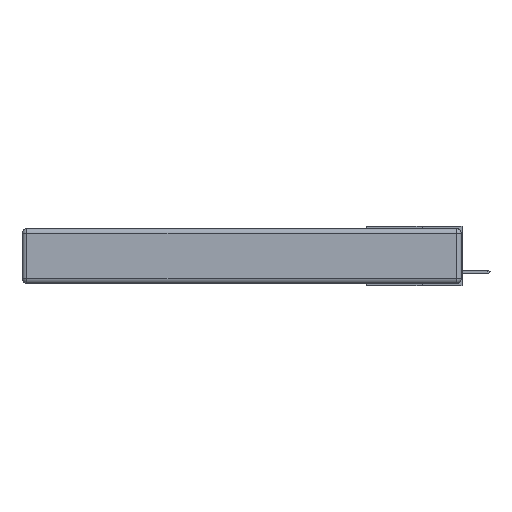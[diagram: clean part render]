
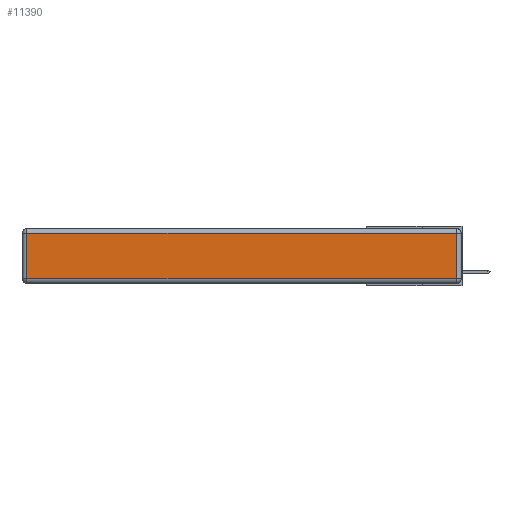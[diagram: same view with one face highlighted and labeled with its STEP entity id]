
A CAD part, left-side view. The second image highlights one B-rep face of the part: STEP entity #11390.
In plain terms, the highlighted planar face has unit normal (-1, 0, 0).
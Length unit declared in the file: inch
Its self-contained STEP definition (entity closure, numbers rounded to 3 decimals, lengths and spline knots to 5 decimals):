
#704 = CARTESIAN_POINT ( 'NONE',  ( 0., 0., -0.313 ) ) ;
#981 = VECTOR ( 'NONE', #4588, 39.37008 ) ;
#1590 = ORIENTED_EDGE ( 'NONE', *, *, #9891, .T. ) ;
#2071 = DIRECTION ( 'NONE',  ( 0., 0., 1. ) ) ;
#2267 = CARTESIAN_POINT ( 'NONE',  ( 0., 0., -0.343 ) ) ;
#2925 = VECTOR ( 'NONE', #2071, 39.37008 ) ;
#3695 = PLANE ( 'NONE',  #12956 ) ;
#4060 = EDGE_CURVE ( 'NONE', #6856, #14150, #15080, .T. ) ;
#4332 = CARTESIAN_POINT ( 'NONE',  ( 0., 0.03, -0.313 ) ) ;
#4337 = VERTEX_POINT ( 'NONE', #4332 ) ;
#4588 = DIRECTION ( 'NONE',  ( 0., 0., -1. ) ) ;
#5303 = DIRECTION ( 'NONE',  ( 0., 1., 0. ) ) ;
#6033 = VERTEX_POINT ( 'NONE', #11285 ) ;
#6305 = CARTESIAN_POINT ( 'NONE',  ( 0., 2.72, -0.343 ) ) ;
#6407 = VECTOR ( 'NONE', #5303, 39.37008 ) ;
#6719 = CARTESIAN_POINT ( 'NONE',  ( 0., 0.03, -0.343 ) ) ;
#6856 = VERTEX_POINT ( 'NONE', #18652 ) ;
#6917 = LINE ( 'NONE', #14931, #6407 ) ;
#8544 = DIRECTION ( 'NONE',  ( -1., 0., 0. ) ) ;
#8622 = EDGE_LOOP ( 'NONE', ( #1590, #11310, #20942, #16307 ) ) ;
#9177 = LINE ( 'NONE', #704, #14847 ) ;
#9891 = EDGE_CURVE ( 'NONE', #14150, #4337, #9177, .T. ) ;
#11285 = CARTESIAN_POINT ( 'NONE',  ( 0., 0.03, -0.03 ) ) ;
#11310 = ORIENTED_EDGE ( 'NONE', *, *, #16631, .T. ) ;
#11390 = ADVANCED_FACE ( 'NONE', ( #17583 ), #3695, .T. ) ;
#11823 = DIRECTION ( 'NONE',  ( 0., 0., 1. ) ) ;
#12956 = AXIS2_PLACEMENT_3D ( 'NONE', #2267, #8544, #11823 ) ;
#14150 = VERTEX_POINT ( 'NONE', #15958 ) ;
#14847 = VECTOR ( 'NONE', #15442, 39.37008 ) ;
#14931 = CARTESIAN_POINT ( 'NONE',  ( 0., 2.75, -0.03 ) ) ;
#15080 = LINE ( 'NONE', #6305, #981 ) ;
#15442 = DIRECTION ( 'NONE',  ( 0., -1., 0. ) ) ;
#15958 = CARTESIAN_POINT ( 'NONE',  ( 0., 2.72, -0.313 ) ) ;
#16307 = ORIENTED_EDGE ( 'NONE', *, *, #4060, .T. ) ;
#16631 = EDGE_CURVE ( 'NONE', #4337, #6033, #18282, .T. ) ;
#17583 = FACE_OUTER_BOUND ( 'NONE', #8622, .T. ) ;
#18282 = LINE ( 'NONE', #6719, #2925 ) ;
#18652 = CARTESIAN_POINT ( 'NONE',  ( 0., 2.72, -0.03 ) ) ;
#18724 = EDGE_CURVE ( 'NONE', #6033, #6856, #6917, .T. ) ;
#20942 = ORIENTED_EDGE ( 'NONE', *, *, #18724, .T. ) ;
